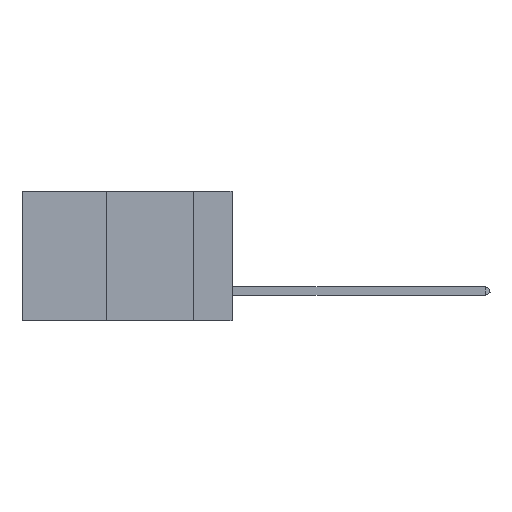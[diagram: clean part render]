
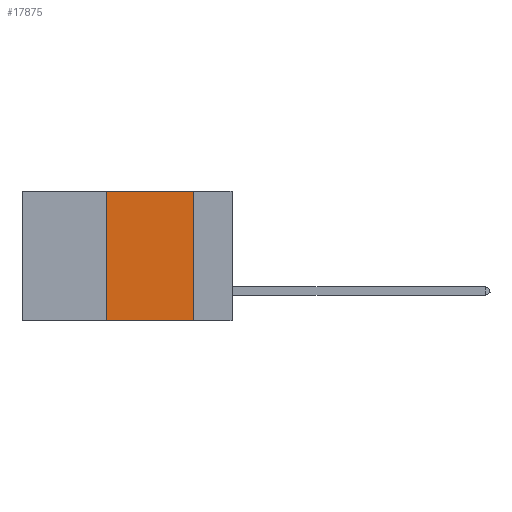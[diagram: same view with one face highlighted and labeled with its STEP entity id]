
A CAD part, left-side view. The second image highlights one B-rep face of the part: STEP entity #17875.
In plain terms, the highlighted planar face has unit normal (-1, 0, 0).
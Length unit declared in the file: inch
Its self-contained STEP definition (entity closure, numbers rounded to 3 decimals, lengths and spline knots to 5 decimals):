
#23 = LINE ( 'NONE', #18500, #2614 ) ;
#447 = CARTESIAN_POINT ( 'NONE',  ( 0., 0.11, -0.37 ) ) ;
#928 = DIRECTION ( 'NONE',  ( 1., 0., 0. ) ) ;
#1907 = DIRECTION ( 'NONE',  ( 0., -1., 0. ) ) ;
#2614 = VECTOR ( 'NONE', #1907, 39.37008 ) ;
#3702 = LINE ( 'NONE', #35468, #34595 ) ;
#3779 = LINE ( 'NONE', #25319, #35138 ) ;
#5469 = EDGE_CURVE ( 'NONE', #31422, #17859, #3779, .T. ) ;
#6291 = DIRECTION ( 'NONE',  ( 0., 0., 1. ) ) ;
#6498 = VERTEX_POINT ( 'NONE', #9304 ) ;
#8547 = CARTESIAN_POINT ( 'NONE',  ( 0., 0.11, 0. ) ) ;
#9304 = CARTESIAN_POINT ( 'NONE',  ( 0., 0.11, 0. ) ) ;
#13241 = DIRECTION ( 'NONE',  ( 0., -1., 0. ) ) ;
#14531 = EDGE_LOOP ( 'NONE', ( #33292, #18471, #25776, #31724 ) ) ;
#15194 = PLANE ( 'NONE',  #23860 ) ;
#16882 = LINE ( 'NONE', #8547, #17774 ) ;
#17774 = VECTOR ( 'NONE', #19701, 39.37008 ) ;
#17859 = VERTEX_POINT ( 'NONE', #30765 ) ;
#17875 = ADVANCED_FACE ( 'NONE', ( #32825 ), #15194, .F. ) ;
#18471 = ORIENTED_EDGE ( 'NONE', *, *, #23548, .F. ) ;
#18500 = CARTESIAN_POINT ( 'NONE',  ( 0., 0.6, 0. ) ) ;
#19701 = DIRECTION ( 'NONE',  ( 0., 0., -1. ) ) ;
#23548 = EDGE_CURVE ( 'NONE', #17859, #6498, #23, .T. ) ;
#23860 = AXIS2_PLACEMENT_3D ( 'NONE', #25862, #928, #29735 ) ;
#25319 = CARTESIAN_POINT ( 'NONE',  ( 0., 0.36, 0. ) ) ;
#25776 = ORIENTED_EDGE ( 'NONE', *, *, #5469, .F. ) ;
#25862 = CARTESIAN_POINT ( 'NONE',  ( 0., 0.6, 0. ) ) ;
#26085 = EDGE_CURVE ( 'NONE', #6498, #28008, #16882, .T. ) ;
#26506 = EDGE_CURVE ( 'NONE', #31422, #28008, #3702, .T. ) ;
#26584 = CARTESIAN_POINT ( 'NONE',  ( 0., 0.36, -0.37 ) ) ;
#28008 = VERTEX_POINT ( 'NONE', #447 ) ;
#29735 = DIRECTION ( 'NONE',  ( 0., 0., -1. ) ) ;
#30765 = CARTESIAN_POINT ( 'NONE',  ( 0., 0.36, 0. ) ) ;
#31422 = VERTEX_POINT ( 'NONE', #26584 ) ;
#31724 = ORIENTED_EDGE ( 'NONE', *, *, #26506, .T. ) ;
#32825 = FACE_OUTER_BOUND ( 'NONE', #14531, .T. ) ;
#33292 = ORIENTED_EDGE ( 'NONE', *, *, #26085, .F. ) ;
#34595 = VECTOR ( 'NONE', #13241, 39.37008 ) ;
#35138 = VECTOR ( 'NONE', #6291, 39.37008 ) ;
#35468 = CARTESIAN_POINT ( 'NONE',  ( 0., 0.6, -0.37 ) ) ;
